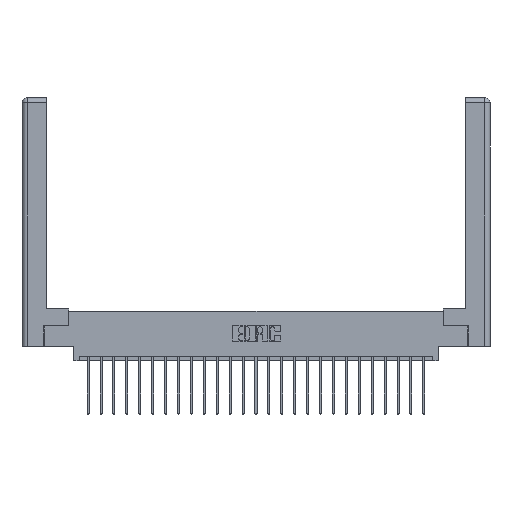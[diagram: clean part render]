
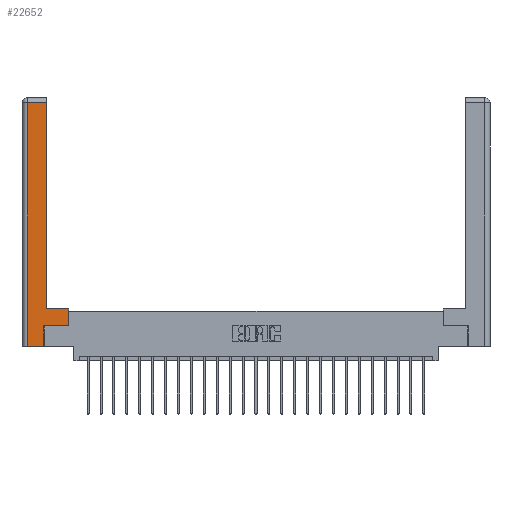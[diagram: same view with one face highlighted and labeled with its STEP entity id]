
A CAD part, top view. The second image highlights one B-rep face of the part: STEP entity #22652.
In plain terms, the highlighted planar face has unit normal (0, 0, 1).
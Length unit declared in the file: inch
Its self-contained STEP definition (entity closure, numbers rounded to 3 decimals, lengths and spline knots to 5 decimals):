
#1157 = CARTESIAN_POINT ( 'NONE',  ( 0.565, 0.245, 0. ) ) ;
#1243 = CARTESIAN_POINT ( 'NONE',  ( 0.565, 0.45, 0. ) ) ;
#1682 = FACE_OUTER_BOUND ( 'NONE', #2559, .T. ) ;
#1696 = AXIS2_PLACEMENT_3D ( 'NONE', #15664, #5548, #7714 ) ;
#2339 = PLANE ( 'NONE',  #1696 ) ;
#2385 = VECTOR ( 'NONE', #17247, 39.37008 ) ;
#2543 = LINE ( 'NONE', #1243, #6272 ) ;
#2559 = EDGE_LOOP ( 'NONE', ( #15399, #9888, #5792, #7827, #21844, #2730, #5236, #23668 ) ) ;
#2730 = ORIENTED_EDGE ( 'NONE', *, *, #7610, .T. ) ;
#3155 = CARTESIAN_POINT ( 'NONE',  ( 0.295, 0.45, 0. ) ) ;
#3502 = CARTESIAN_POINT ( 'NONE',  ( 0.265, 0., 0. ) ) ;
#4419 = VERTEX_POINT ( 'NONE', #16275 ) ;
#4630 = VECTOR ( 'NONE', #11334, 39.37008 ) ;
#4708 = EDGE_CURVE ( 'NONE', #7868, #10894, #13126, .T. ) ;
#4888 = DIRECTION ( 'NONE',  ( 0., 1., 0. ) ) ;
#5236 = ORIENTED_EDGE ( 'NONE', *, *, #23739, .T. ) ;
#5491 = EDGE_CURVE ( 'NONE', #20276, #17475, #18029, .T. ) ;
#5548 = DIRECTION ( 'NONE',  ( 0., 0., -1. ) ) ;
#5792 = ORIENTED_EDGE ( 'NONE', *, *, #9506, .T. ) ;
#6208 = LINE ( 'NONE', #16692, #16180 ) ;
#6272 = VECTOR ( 'NONE', #4888, 39.37008 ) ;
#7208 = CARTESIAN_POINT ( 'NONE',  ( 0.265, 0., 0. ) ) ;
#7561 = LINE ( 'NONE', #9365, #18142 ) ;
#7610 = EDGE_CURVE ( 'NONE', #10894, #10779, #19165, .T. ) ;
#7714 = DIRECTION ( 'NONE',  ( -1., 0., 0. ) ) ;
#7827 = ORIENTED_EDGE ( 'NONE', *, *, #14157, .T. ) ;
#7868 = VERTEX_POINT ( 'NONE', #7208 ) ;
#7961 = VERTEX_POINT ( 'NONE', #19605 ) ;
#8259 = CARTESIAN_POINT ( 'NONE',  ( 0.0615, 0., 0. ) ) ;
#9002 = VECTOR ( 'NONE', #9162, 39.37008 ) ;
#9077 = DIRECTION ( 'NONE',  ( 0., 1., 0. ) ) ;
#9162 = DIRECTION ( 'NONE',  ( -1., 0., 0. ) ) ;
#9365 = CARTESIAN_POINT ( 'NONE',  ( 0.295, 3., 0. ) ) ;
#9462 = DIRECTION ( 'NONE',  ( 0., 1., 0. ) ) ;
#9506 = EDGE_CURVE ( 'NONE', #4419, #7961, #10369, .T. ) ;
#9508 = CARTESIAN_POINT ( 'NONE',  ( 0.265, 0.245, 0. ) ) ;
#9888 = ORIENTED_EDGE ( 'NONE', *, *, #25556, .T. ) ;
#10369 = LINE ( 'NONE', #8259, #16285 ) ;
#10428 = VERTEX_POINT ( 'NONE', #19517 ) ;
#10669 = CARTESIAN_POINT ( 'NONE',  ( 0.565, 0.45, 0. ) ) ;
#10779 = VERTEX_POINT ( 'NONE', #1157 ) ;
#10894 = VERTEX_POINT ( 'NONE', #9508 ) ;
#11334 = DIRECTION ( 'NONE',  ( 1., 0., 0. ) ) ;
#13126 = LINE ( 'NONE', #20828, #24545 ) ;
#14157 = EDGE_CURVE ( 'NONE', #7961, #7868, #22977, .T. ) ;
#14940 = CARTESIAN_POINT ( 'NONE',  ( 0.565, 0.245, 0. ) ) ;
#15399 = ORIENTED_EDGE ( 'NONE', *, *, #23091, .T. ) ;
#15664 = CARTESIAN_POINT ( 'NONE',  ( 0., 0., 0. ) ) ;
#16180 = VECTOR ( 'NONE', #24016, 39.37008 ) ;
#16275 = CARTESIAN_POINT ( 'NONE',  ( 0.0615, 2.94, 0. ) ) ;
#16285 = VECTOR ( 'NONE', #16344, 39.37008 ) ;
#16344 = DIRECTION ( 'NONE',  ( 0., -1., 0. ) ) ;
#16692 = CARTESIAN_POINT ( 'NONE',  ( 0.0615, 2.94, 0. ) ) ;
#17247 = DIRECTION ( 'NONE',  ( 1., 0., 0. ) ) ;
#17475 = VERTEX_POINT ( 'NONE', #3155 ) ;
#18029 = LINE ( 'NONE', #22782, #9002 ) ;
#18142 = VECTOR ( 'NONE', #9462, 39.37008 ) ;
#19165 = LINE ( 'NONE', #14940, #2385 ) ;
#19517 = CARTESIAN_POINT ( 'NONE',  ( 0.295, 2.94, 0. ) ) ;
#19605 = CARTESIAN_POINT ( 'NONE',  ( 0.0615, 0., 0. ) ) ;
#20276 = VERTEX_POINT ( 'NONE', #10669 ) ;
#20828 = CARTESIAN_POINT ( 'NONE',  ( 0.265, 0.245, 0. ) ) ;
#21844 = ORIENTED_EDGE ( 'NONE', *, *, #4708, .T. ) ;
#22652 = ADVANCED_FACE ( 'NONE', ( #1682 ), #2339, .F. ) ;
#22782 = CARTESIAN_POINT ( 'NONE',  ( 0.295, 0.45, 0. ) ) ;
#22977 = LINE ( 'NONE', #3502, #4630 ) ;
#23091 = EDGE_CURVE ( 'NONE', #17475, #10428, #7561, .T. ) ;
#23668 = ORIENTED_EDGE ( 'NONE', *, *, #5491, .T. ) ;
#23739 = EDGE_CURVE ( 'NONE', #10779, #20276, #2543, .T. ) ;
#24016 = DIRECTION ( 'NONE',  ( -1., 0., 0. ) ) ;
#24545 = VECTOR ( 'NONE', #9077, 39.37008 ) ;
#25556 = EDGE_CURVE ( 'NONE', #10428, #4419, #6208, .T. ) ;
